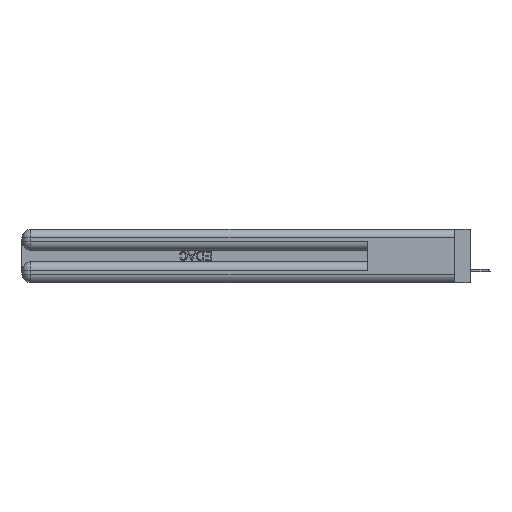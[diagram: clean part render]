
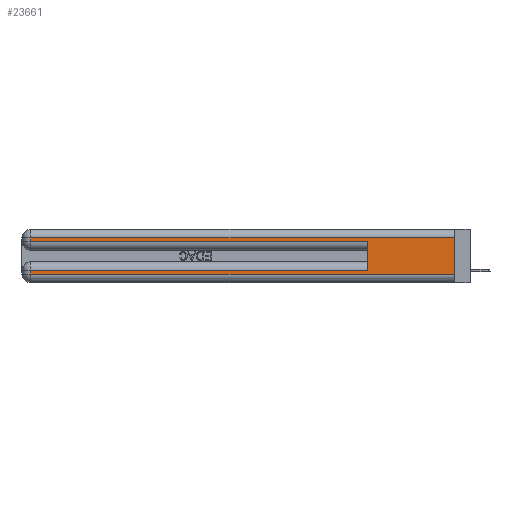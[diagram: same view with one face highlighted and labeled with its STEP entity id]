
A CAD part, left-side view. The second image highlights one B-rep face of the part: STEP entity #23661.
In plain terms, the highlighted planar face has unit normal (-1, 0, 0).
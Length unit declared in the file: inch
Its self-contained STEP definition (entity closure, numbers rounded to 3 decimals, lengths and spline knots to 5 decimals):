
#472 = VERTEX_POINT ( 'NONE', #1914 ) ;
#1323 = EDGE_CURVE ( 'NONE', #41799, #41496, #16621, .T. ) ;
#1587 = VECTOR ( 'NONE', #12736, 39.37008 ) ;
#1601 = EDGE_CURVE ( 'NONE', #46529, #31427, #40121, .T. ) ;
#1797 = VECTOR ( 'NONE', #44108, 39.37008 ) ;
#1914 = CARTESIAN_POINT ( 'NONE',  ( 0., 2.94, 0.31 ) ) ;
#2668 = CARTESIAN_POINT ( 'NONE',  ( 0., 0., 0.31 ) ) ;
#3227 = ORIENTED_EDGE ( 'NONE', *, *, #3728, .T. ) ;
#3333 = DIRECTION ( 'NONE',  ( 0., 0., -1. ) ) ;
#3345 = ORIENTED_EDGE ( 'NONE', *, *, #1601, .T. ) ;
#3728 = EDGE_CURVE ( 'NONE', #25890, #41496, #29005, .T. ) ;
#4156 = EDGE_LOOP ( 'NONE', ( #15109, #18549, #23625, #3227, #26721, #32562, #45638, #3345 ) ) ;
#6077 = LINE ( 'NONE', #10656, #42480 ) ;
#6550 = DIRECTION ( 'NONE',  ( 0., 0., -1. ) ) ;
#8485 = EDGE_CURVE ( 'NONE', #30896, #472, #28481, .T. ) ;
#9306 = CARTESIAN_POINT ( 'NONE',  ( 0., 0.6, 0.085 ) ) ;
#9968 = CARTESIAN_POINT ( 'NONE',  ( 0., 2.94, 0.085 ) ) ;
#10656 = CARTESIAN_POINT ( 'NONE',  ( 0., 2.94, 0.37 ) ) ;
#11658 = CARTESIAN_POINT ( 'NONE',  ( 0., 0., 0.37 ) ) ;
#12035 = CARTESIAN_POINT ( 'NONE',  ( 0., 2.94, 0.37 ) ) ;
#12736 = DIRECTION ( 'NONE',  ( 0., 0., 1. ) ) ;
#15109 = ORIENTED_EDGE ( 'NONE', *, *, #42426, .F. ) ;
#15129 = EDGE_CURVE ( 'NONE', #18007, #46529, #6077, .T. ) ;
#15428 = LINE ( 'NONE', #12035, #47244 ) ;
#16034 = AXIS2_PLACEMENT_3D ( 'NONE', #40334, #47640, #3333 ) ;
#16621 = LINE ( 'NONE', #28086, #1587 ) ;
#17804 = CARTESIAN_POINT ( 'NONE',  ( 0., 0., 0.31 ) ) ;
#18007 = VERTEX_POINT ( 'NONE', #9968 ) ;
#18179 = PLANE ( 'NONE',  #16034 ) ;
#18549 = ORIENTED_EDGE ( 'NONE', *, *, #8485, .T. ) ;
#18728 = DIRECTION ( 'NONE',  ( 0., 0., -1. ) ) ;
#20366 = VECTOR ( 'NONE', #46487, 39.37008 ) ;
#20915 = LINE ( 'NONE', #39421, #20366 ) ;
#21141 = DIRECTION ( 'NONE',  ( 0., -1., 0. ) ) ;
#21307 = CARTESIAN_POINT ( 'NONE',  ( 0., 0.6, 0.285 ) ) ;
#23625 = ORIENTED_EDGE ( 'NONE', *, *, #26939, .T. ) ;
#23661 = ADVANCED_FACE ( 'NONE', ( #39388 ), #18179, .F. ) ;
#24209 = VECTOR ( 'NONE', #21141, 39.37008 ) ;
#24673 = VECTOR ( 'NONE', #18728, 39.37008 ) ;
#25890 = VERTEX_POINT ( 'NONE', #28551 ) ;
#26079 = LINE ( 'NONE', #11658, #24673 ) ;
#26721 = ORIENTED_EDGE ( 'NONE', *, *, #1323, .F. ) ;
#26939 = EDGE_CURVE ( 'NONE', #472, #25890, #15428, .T. ) ;
#28002 = DIRECTION ( 'NONE',  ( 0., 1., 0. ) ) ;
#28086 = CARTESIAN_POINT ( 'NONE',  ( 0., 0.6, 0.145 ) ) ;
#28481 = LINE ( 'NONE', #2668, #45044 ) ;
#28551 = CARTESIAN_POINT ( 'NONE',  ( 0., 2.94, 0.285 ) ) ;
#29005 = LINE ( 'NONE', #43871, #1797 ) ;
#30667 = EDGE_CURVE ( 'NONE', #41799, #18007, #20915, .T. ) ;
#30896 = VERTEX_POINT ( 'NONE', #17804 ) ;
#31427 = VERTEX_POINT ( 'NONE', #44542 ) ;
#31623 = CARTESIAN_POINT ( 'NONE',  ( 0., 2.94, 0.06 ) ) ;
#32562 = ORIENTED_EDGE ( 'NONE', *, *, #30667, .T. ) ;
#38117 = DIRECTION ( 'NONE',  ( 0., 0., -1. ) ) ;
#39388 = FACE_OUTER_BOUND ( 'NONE', #4156, .T. ) ;
#39413 = CARTESIAN_POINT ( 'NONE',  ( 0., 0., 0.06 ) ) ;
#39421 = CARTESIAN_POINT ( 'NONE',  ( 0., 0., 0.085 ) ) ;
#40121 = LINE ( 'NONE', #39413, #24209 ) ;
#40334 = CARTESIAN_POINT ( 'NONE',  ( 0., 0., 0.37 ) ) ;
#41496 = VERTEX_POINT ( 'NONE', #21307 ) ;
#41799 = VERTEX_POINT ( 'NONE', #9306 ) ;
#42426 = EDGE_CURVE ( 'NONE', #30896, #31427, #26079, .T. ) ;
#42480 = VECTOR ( 'NONE', #6550, 39.37008 ) ;
#43871 = CARTESIAN_POINT ( 'NONE',  ( 0., 0., 0.285 ) ) ;
#44108 = DIRECTION ( 'NONE',  ( 0., -1., 0. ) ) ;
#44542 = CARTESIAN_POINT ( 'NONE',  ( 0., 0., 0.06 ) ) ;
#45044 = VECTOR ( 'NONE', #28002, 39.37008 ) ;
#45638 = ORIENTED_EDGE ( 'NONE', *, *, #15129, .T. ) ;
#46487 = DIRECTION ( 'NONE',  ( 0., 1., 0. ) ) ;
#46529 = VERTEX_POINT ( 'NONE', #31623 ) ;
#47244 = VECTOR ( 'NONE', #38117, 39.37008 ) ;
#47640 = DIRECTION ( 'NONE',  ( 1., 0., 0. ) ) ;
